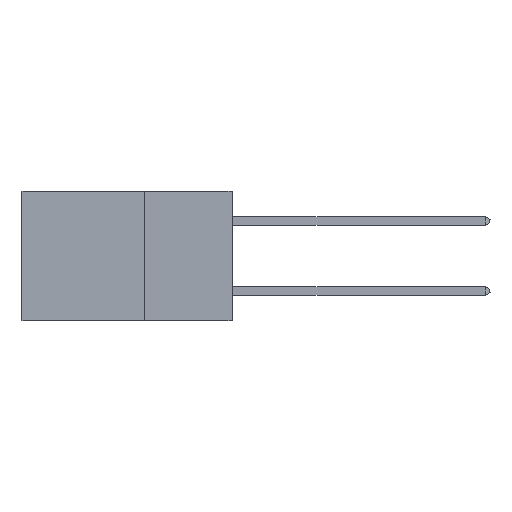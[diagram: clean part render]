
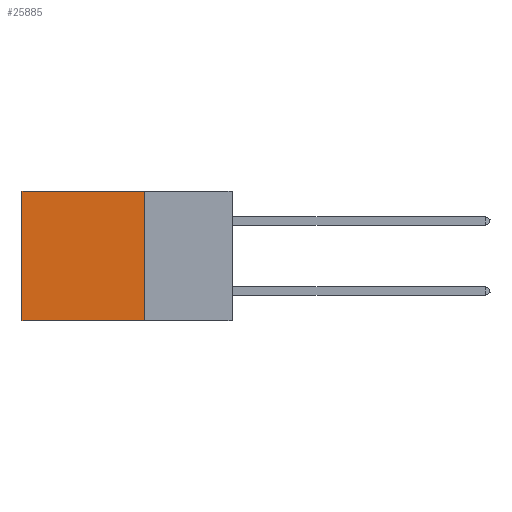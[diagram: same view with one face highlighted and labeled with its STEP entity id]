
A CAD part, left-side view. The second image highlights one B-rep face of the part: STEP entity #25885.
In plain terms, the highlighted planar face has unit normal (-1, 0, 0).
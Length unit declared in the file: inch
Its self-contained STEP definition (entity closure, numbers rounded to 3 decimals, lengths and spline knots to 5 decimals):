
#332 = CARTESIAN_POINT ( 'NONE',  ( 0.2875, 0.6, 0. ) ) ;
#858 = DIRECTION ( 'NONE',  ( 0., 1., 0. ) ) ;
#912 = EDGE_CURVE ( 'NONE', #27074, #3942, #29357, .T. ) ;
#1288 = CARTESIAN_POINT ( 'NONE',  ( 0.2875, 0.25, 0. ) ) ;
#3223 = VERTEX_POINT ( 'NONE', #1288 ) ;
#3942 = VERTEX_POINT ( 'NONE', #9374 ) ;
#3953 = ORIENTED_EDGE ( 'NONE', *, *, #912, .F. ) ;
#4263 = DIRECTION ( 'NONE',  ( 1., 0., 0. ) ) ;
#5703 = DIRECTION ( 'NONE',  ( 0., 0., -1. ) ) ;
#6241 = LINE ( 'NONE', #332, #13331 ) ;
#7461 = EDGE_CURVE ( 'NONE', #3223, #32644, #32468, .T. ) ;
#8279 = ORIENTED_EDGE ( 'NONE', *, *, #13665, .F. ) ;
#8943 = CARTESIAN_POINT ( 'NONE',  ( 0.2875, 0.25, -0.37 ) ) ;
#9374 = CARTESIAN_POINT ( 'NONE',  ( 0.2875, 0.6, -0.37 ) ) ;
#10452 = EDGE_LOOP ( 'NONE', ( #31157, #3953, #8279, #15883 ) ) ;
#11130 = AXIS2_PLACEMENT_3D ( 'NONE', #20186, #4263, #22824 ) ;
#12178 = FACE_OUTER_BOUND ( 'NONE', #10452, .T. ) ;
#13331 = VECTOR ( 'NONE', #5703, 39.37008 ) ;
#13395 = LINE ( 'NONE', #31242, #27403 ) ;
#13665 = EDGE_CURVE ( 'NONE', #3223, #27074, #13395, .T. ) ;
#14532 = VECTOR ( 'NONE', #19042, 39.37008 ) ;
#14839 = PLANE ( 'NONE',  #11130 ) ;
#15551 = DIRECTION ( 'NONE',  ( 0., 0., -1. ) ) ;
#15883 = ORIENTED_EDGE ( 'NONE', *, *, #7461, .T. ) ;
#16804 = CARTESIAN_POINT ( 'NONE',  ( 0.2875, 0.25, 0. ) ) ;
#19042 = DIRECTION ( 'NONE',  ( 0., 1., 0. ) ) ;
#19065 = EDGE_CURVE ( 'NONE', #32644, #3942, #6241, .T. ) ;
#20186 = CARTESIAN_POINT ( 'NONE',  ( 0.2875, 0.25, 0. ) ) ;
#22824 = DIRECTION ( 'NONE',  ( 0., 0., -1. ) ) ;
#25885 = ADVANCED_FACE ( 'NONE', ( #12178 ), #14839, .F. ) ;
#26398 = VECTOR ( 'NONE', #858, 39.37008 ) ;
#27074 = VERTEX_POINT ( 'NONE', #8943 ) ;
#27403 = VECTOR ( 'NONE', #15551, 39.37008 ) ;
#29357 = LINE ( 'NONE', #33936, #14532 ) ;
#31157 = ORIENTED_EDGE ( 'NONE', *, *, #19065, .T. ) ;
#31242 = CARTESIAN_POINT ( 'NONE',  ( 0.2875, 0.25, 0. ) ) ;
#32468 = LINE ( 'NONE', #16804, #26398 ) ;
#32644 = VERTEX_POINT ( 'NONE', #33809 ) ;
#33809 = CARTESIAN_POINT ( 'NONE',  ( 0.2875, 0.6, 0. ) ) ;
#33936 = CARTESIAN_POINT ( 'NONE',  ( 0.2875, 0.25, -0.37 ) ) ;
